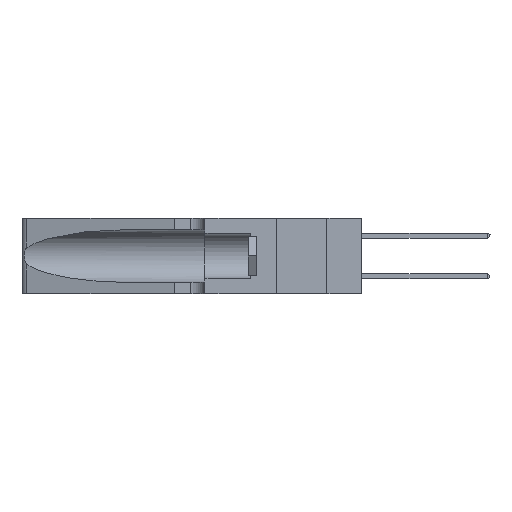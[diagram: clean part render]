
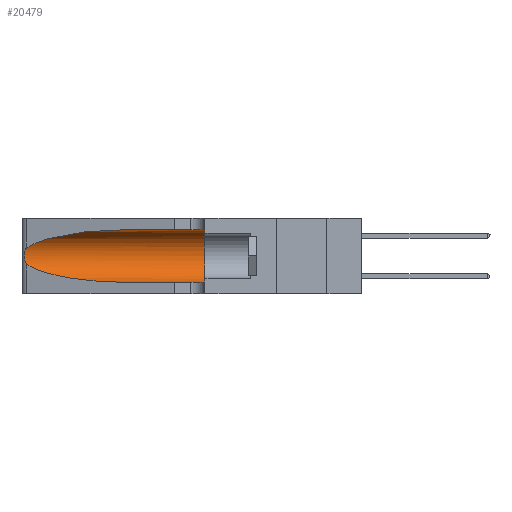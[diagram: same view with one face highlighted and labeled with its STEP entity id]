
A CAD part, left-side view. The second image highlights one B-rep face of the part: STEP entity #20479.
In plain terms, the highlighted cylindrical face has radius 3.308 mm (diameter 6.617 mm), a partial arc.
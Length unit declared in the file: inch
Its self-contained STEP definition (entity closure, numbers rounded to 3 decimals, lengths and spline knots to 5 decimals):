
#553 = DIRECTION ( 'NONE',  ( 0., -1., 0. ) ) ;
#697 = EDGE_CURVE ( 'NONE', #20039, #9052, #38464, .T. ) ;
#864 = CARTESIAN_POINT ( 'NONE',  ( 0.26075, 1.23896, 0.19203 ) ) ;
#2122 =( BOUNDED_CURVE ( )  B_SPLINE_CURVE ( 3, ( #36764, #22459, #29827, #32839 ),
 .UNSPECIFIED., .F., .F. ) 
 B_SPLINE_CURVE_WITH_KNOTS ( ( 4, 4 ),
 ( 3.44316, 4.71239 ),
 .UNSPECIFIED. ) 
 CURVE ( )  GEOMETRIC_REPRESENTATION_ITEM ( )  RATIONAL_B_SPLINE_CURVE ( ( 1., 0.87, 0.87, 1. ) ) 
 REPRESENTATION_ITEM ( '' )  );
#2375 = EDGE_CURVE ( 'NONE', #15232, #22423, #43706, .T. ) ;
#3572 = DIRECTION ( 'NONE',  ( 0., 0., 1. ) ) ;
#4464 = CARTESIAN_POINT ( 'NONE',  ( 0.25789, 1.23486, 0.15765 ) ) ;
#4637 = CARTESIAN_POINT ( 'NONE',  ( 0.1305, 1.61858, 0.05475 ) ) ;
#5275 = CARTESIAN_POINT ( 'NONE',  ( 0.1305, 0.72297, 0.05475 ) ) ;
#5948 = ORIENTED_EDGE ( 'NONE', *, *, #32006, .F. ) ;
#7195 = CARTESIAN_POINT ( 'NONE',  ( 0.1305, 0.35, 0.185 ) ) ;
#8426 = CARTESIAN_POINT ( 'NONE',  ( 0.25487, 1.22718, 0.22369 ) ) ;
#8573 = CARTESIAN_POINT ( 'NONE',  ( 0.25639, 1.23186, 0.15144 ) ) ;
#9052 = VERTEX_POINT ( 'NONE', #9563 ) ;
#9350 = CARTESIAN_POINT ( 'NONE',  ( 0.26018, 1.23835, 0.19895 ) ) ;
#9563 = CARTESIAN_POINT ( 'NONE',  ( 0.1305, 0.35, 0.05475 ) ) ;
#10235 = CYLINDRICAL_SURFACE ( 'NONE', #16705, 0.13025 ) ;
#11509 = CARTESIAN_POINT ( 'NONE',  ( 0.26075, 1.23896, 0.178 ) ) ;
#11938 = ORIENTED_EDGE ( 'NONE', *, *, #2375, .T. ) ;
#12538 = CARTESIAN_POINT ( 'NONE',  ( 0.1305, 0.35, 0.31525 ) ) ;
#12665 = EDGE_LOOP ( 'NONE', ( #11938, #44642, #30976, #24367, #29230, #5948 ) ) ;
#15232 = VERTEX_POINT ( 'NONE', #23605 ) ;
#16367 = CARTESIAN_POINT ( 'NONE',  ( 0.2373, 1.15595, 0.28018 ) ) ;
#16705 = AXIS2_PLACEMENT_3D ( 'NONE', #37363, #33760, #19485 ) ;
#17319 = B_SPLINE_CURVE_WITH_KNOTS ( 'NONE', 3,
 ( #8426, #43736, #19032, #19335, #43882, #9350, #864, #11509, #18704, #25913, #4464, #8573, #33307, #33628 ),
 .UNSPECIFIED., .F., .F.,
 ( 4, 2, 2, 2, 2, 2, 4 ),
 ( 0., 0.00027, 0.00053, 0.00107, 0.0016, 0.00187, 0.00214 ),
 .UNSPECIFIED. ) ;
#17514 = EDGE_CURVE ( 'NONE', #32835, #9052, #19970, .T. ) ;
#18704 = CARTESIAN_POINT ( 'NONE',  ( 0.26017, 1.23833, 0.17102 ) ) ;
#19032 = CARTESIAN_POINT ( 'NONE',  ( 0.25639, 1.23184, 0.21858 ) ) ;
#19335 = CARTESIAN_POINT ( 'NONE',  ( 0.25787, 1.23484, 0.2124 ) ) ;
#19342 = CARTESIAN_POINT ( 'NONE',  ( 0.18966, 0.96281, 0.31525 ) ) ;
#19485 = DIRECTION ( 'NONE',  ( 0., 0., -1. ) ) ;
#19597 = LINE ( 'NONE', #29508, #22357 ) ;
#19970 = CIRCLE ( 'NONE', #39433, 0.13025 ) ;
#20039 = VERTEX_POINT ( 'NONE', #5275 ) ;
#20219 = CARTESIAN_POINT ( 'NONE',  ( 0.25487, 1.22718, 0.22369 ) ) ;
#20479 = ADVANCED_FACE ( 'NONE', ( #21989 ), #10235, .F. ) ;
#21989 = FACE_OUTER_BOUND ( 'NONE', #12665, .T. ) ;
#22357 = VECTOR ( 'NONE', #553, 39.37008 ) ;
#22423 = VERTEX_POINT ( 'NONE', #20219 ) ;
#22459 = CARTESIAN_POINT ( 'NONE',  ( 0.2373, 1.15595, 0.08982 ) ) ;
#23605 = CARTESIAN_POINT ( 'NONE',  ( 0.1305, 0.72297, 0.31525 ) ) ;
#24367 = ORIENTED_EDGE ( 'NONE', *, *, #697, .T. ) ;
#25913 = CARTESIAN_POINT ( 'NONE',  ( 0.25856, 1.23593, 0.16098 ) ) ;
#29230 = ORIENTED_EDGE ( 'NONE', *, *, #17514, .F. ) ;
#29508 = CARTESIAN_POINT ( 'NONE',  ( 0.1305, 1.61858, 0.31525 ) ) ;
#29827 = CARTESIAN_POINT ( 'NONE',  ( 0.18966, 0.96281, 0.05475 ) ) ;
#30976 = ORIENTED_EDGE ( 'NONE', *, *, #32034, .T. ) ;
#32006 = EDGE_CURVE ( 'NONE', #15232, #32835, #19597, .T. ) ;
#32034 = EDGE_CURVE ( 'NONE', #43583, #20039, #2122, .T. ) ;
#32835 = VERTEX_POINT ( 'NONE', #12538 ) ;
#32839 = CARTESIAN_POINT ( 'NONE',  ( 0.1305, 0.72297, 0.05475 ) ) ;
#33307 = CARTESIAN_POINT ( 'NONE',  ( 0.25555, 1.22993, 0.14849 ) ) ;
#33628 = CARTESIAN_POINT ( 'NONE',  ( 0.25487, 1.22718, 0.14631 ) ) ;
#33760 = DIRECTION ( 'NONE',  ( 0., -1., 0. ) ) ;
#34563 = DIRECTION ( 'NONE',  ( 0., -1., 0. ) ) ;
#36490 = DIRECTION ( 'NONE',  ( 0., 1., 0. ) ) ;
#36764 = CARTESIAN_POINT ( 'NONE',  ( 0.25487, 1.22718, 0.14631 ) ) ;
#37362 = VECTOR ( 'NONE', #34563, 39.37008 ) ;
#37363 = CARTESIAN_POINT ( 'NONE',  ( 0.1305, 1.61858, 0.185 ) ) ;
#38464 = LINE ( 'NONE', #4637, #37362 ) ;
#39433 = AXIS2_PLACEMENT_3D ( 'NONE', #7195, #36490, #3572 ) ;
#40812 = CARTESIAN_POINT ( 'NONE',  ( 0.1305, 0.72297, 0.31525 ) ) ;
#43583 = VERTEX_POINT ( 'NONE', #45958 ) ;
#43706 =( BOUNDED_CURVE ( )  B_SPLINE_CURVE ( 3, ( #40812, #19342, #16367, #44353 ),
 .UNSPECIFIED., .F., .F. ) 
 B_SPLINE_CURVE_WITH_KNOTS ( ( 4, 4 ),
 ( 1.5708, 2.84003 ),
 .UNSPECIFIED. ) 
 CURVE ( )  GEOMETRIC_REPRESENTATION_ITEM ( )  RATIONAL_B_SPLINE_CURVE ( ( 1., 0.87, 0.87, 1. ) ) 
 REPRESENTATION_ITEM ( '' )  );
#43736 = CARTESIAN_POINT ( 'NONE',  ( 0.25555, 1.22994, 0.2215 ) ) ;
#43882 = CARTESIAN_POINT ( 'NONE',  ( 0.25854, 1.2359, 0.20912 ) ) ;
#44353 = CARTESIAN_POINT ( 'NONE',  ( 0.25487, 1.22718, 0.22369 ) ) ;
#44642 = ORIENTED_EDGE ( 'NONE', *, *, #45895, .T. ) ;
#45895 = EDGE_CURVE ( 'NONE', #22423, #43583, #17319, .T. ) ;
#45958 = CARTESIAN_POINT ( 'NONE',  ( 0.25487, 1.22718, 0.14631 ) ) ;
